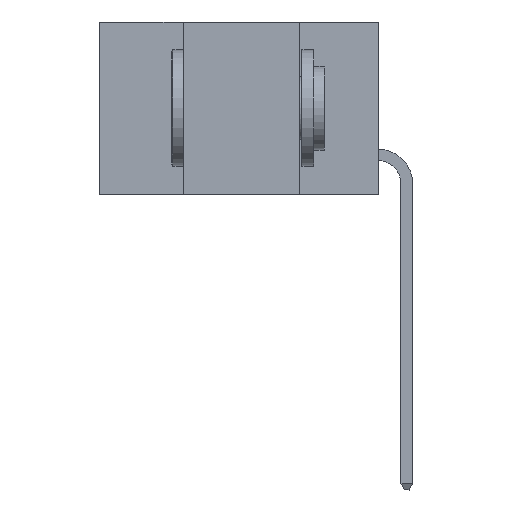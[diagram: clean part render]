
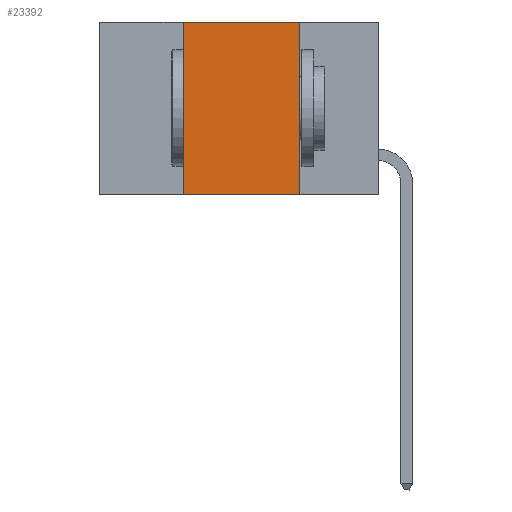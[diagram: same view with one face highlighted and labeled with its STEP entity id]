
A CAD part, left-side view. The second image highlights one B-rep face of the part: STEP entity #23392.
In plain terms, the highlighted planar face has unit normal (-1, 0, 0).
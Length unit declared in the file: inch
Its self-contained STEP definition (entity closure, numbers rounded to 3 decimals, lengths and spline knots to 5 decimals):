
#822 = LINE ( 'NONE', #2865, #12273 ) ;
#1145 = VERTEX_POINT ( 'NONE', #17688 ) ;
#2553 = LINE ( 'NONE', #7621, #22249 ) ;
#2865 = CARTESIAN_POINT ( 'NONE',  ( 0., 0.17, 0. ) ) ;
#3608 = PLANE ( 'NONE',  #22196 ) ;
#4265 = ORIENTED_EDGE ( 'NONE', *, *, #21081, .F. ) ;
#5131 = ORIENTED_EDGE ( 'NONE', *, *, #26463, .F. ) ;
#7030 = DIRECTION ( 'NONE',  ( 0., 0., -1. ) ) ;
#7621 = CARTESIAN_POINT ( 'NONE',  ( 0., 0.6, -0.37 ) ) ;
#7974 = LINE ( 'NONE', #10945, #15184 ) ;
#8266 = CARTESIAN_POINT ( 'NONE',  ( 0., 0.42, 0. ) ) ;
#9895 = CARTESIAN_POINT ( 'NONE',  ( 0., 0.17, -0.37 ) ) ;
#10945 = CARTESIAN_POINT ( 'NONE',  ( 0., 0.42, 0. ) ) ;
#11454 = ORIENTED_EDGE ( 'NONE', *, *, #20212, .T. ) ;
#11691 = VERTEX_POINT ( 'NONE', #23049 ) ;
#12273 = VECTOR ( 'NONE', #7030, 39.37008 ) ;
#12530 = FACE_OUTER_BOUND ( 'NONE', #26428, .T. ) ;
#14013 = DIRECTION ( 'NONE',  ( 0., -1., 0. ) ) ;
#14443 = VERTEX_POINT ( 'NONE', #8266 ) ;
#14869 = ORIENTED_EDGE ( 'NONE', *, *, #26902, .F. ) ;
#15184 = VECTOR ( 'NONE', #24138, 39.37008 ) ;
#15261 = VERTEX_POINT ( 'NONE', #9895 ) ;
#15918 = DIRECTION ( 'NONE',  ( 0., -1., 0. ) ) ;
#16137 = VECTOR ( 'NONE', #15918, 39.37008 ) ;
#17688 = CARTESIAN_POINT ( 'NONE',  ( 0., 0.17, 0. ) ) ;
#18283 = DIRECTION ( 'NONE',  ( 0., 0., -1. ) ) ;
#18560 = CARTESIAN_POINT ( 'NONE',  ( 0., 0.6, 0. ) ) ;
#20212 = EDGE_CURVE ( 'NONE', #11691, #15261, #2553, .T. ) ;
#21081 = EDGE_CURVE ( 'NONE', #1145, #15261, #822, .T. ) ;
#22196 = AXIS2_PLACEMENT_3D ( 'NONE', #18560, #27000, #18283 ) ;
#22249 = VECTOR ( 'NONE', #14013, 39.37008 ) ;
#22369 = CARTESIAN_POINT ( 'NONE',  ( 0., 0.6, 0. ) ) ;
#23049 = CARTESIAN_POINT ( 'NONE',  ( 0., 0.42, -0.37 ) ) ;
#23392 = ADVANCED_FACE ( 'NONE', ( #12530 ), #3608, .F. ) ;
#24138 = DIRECTION ( 'NONE',  ( 0., 0., 1. ) ) ;
#26428 = EDGE_LOOP ( 'NONE', ( #4265, #5131, #14869, #11454 ) ) ;
#26463 = EDGE_CURVE ( 'NONE', #14443, #1145, #26671, .T. ) ;
#26671 = LINE ( 'NONE', #22369, #16137 ) ;
#26902 = EDGE_CURVE ( 'NONE', #11691, #14443, #7974, .T. ) ;
#27000 = DIRECTION ( 'NONE',  ( 1., 0., 0. ) ) ;
